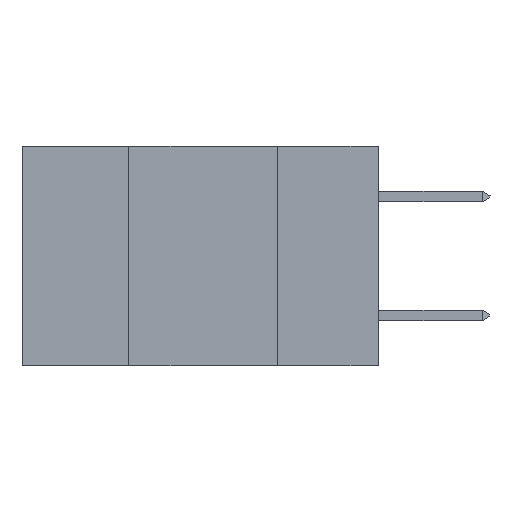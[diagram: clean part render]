
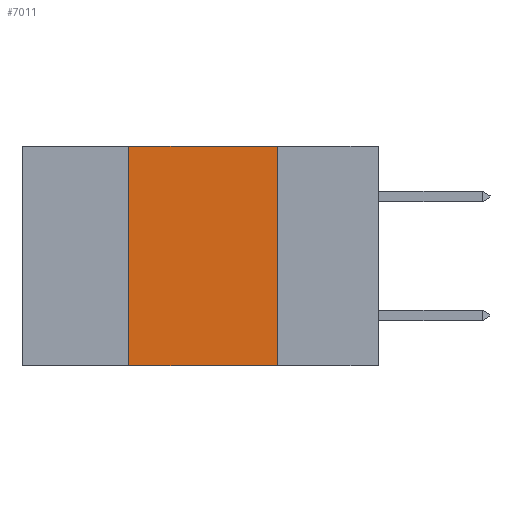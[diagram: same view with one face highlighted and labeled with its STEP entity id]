
A CAD part, left-side view. The second image highlights one B-rep face of the part: STEP entity #7011.
In plain terms, the highlighted planar face has unit normal (-1, 0, 0).
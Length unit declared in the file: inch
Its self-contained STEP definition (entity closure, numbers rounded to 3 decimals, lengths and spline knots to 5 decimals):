
#756 = CARTESIAN_POINT ( 'NONE',  ( 0., 0.17, 0. ) ) ;
#843 = AXIS2_PLACEMENT_3D ( 'NONE', #12461, #4452, #17508 ) ;
#1350 = LINE ( 'NONE', #20598, #4529 ) ;
#2626 = ORIENTED_EDGE ( 'NONE', *, *, #4256, .F. ) ;
#3302 = CARTESIAN_POINT ( 'NONE',  ( 0., 0.17, -0.37 ) ) ;
#3910 = VERTEX_POINT ( 'NONE', #6780 ) ;
#4190 = CARTESIAN_POINT ( 'NONE',  ( 0., 0.6, 0. ) ) ;
#4256 = EDGE_CURVE ( 'NONE', #8670, #11378, #6463, .T. ) ;
#4452 = DIRECTION ( 'NONE',  ( 1., 0., 0. ) ) ;
#4529 = VECTOR ( 'NONE', #16399, 39.37008 ) ;
#4582 = CARTESIAN_POINT ( 'NONE',  ( 0., 0.17, -0.37 ) ) ;
#5583 = DIRECTION ( 'NONE',  ( 0., -1., 0. ) ) ;
#6463 = LINE ( 'NONE', #3302, #13963 ) ;
#6780 = CARTESIAN_POINT ( 'NONE',  ( 0., 0.42, -0.37 ) ) ;
#7011 = ADVANCED_FACE ( 'NONE', ( #15941 ), #10862, .F. ) ;
#7565 = ORIENTED_EDGE ( 'NONE', *, *, #10920, .F. ) ;
#8507 = LINE ( 'NONE', #8926, #17499 ) ;
#8670 = VERTEX_POINT ( 'NONE', #756 ) ;
#8926 = CARTESIAN_POINT ( 'NONE',  ( 0., 0.6, -0.37 ) ) ;
#10862 = PLANE ( 'NONE',  #843 ) ;
#10920 = EDGE_CURVE ( 'NONE', #3910, #11398, #1350, .T. ) ;
#11055 = ORIENTED_EDGE ( 'NONE', *, *, #16998, .F. ) ;
#11378 = VERTEX_POINT ( 'NONE', #4582 ) ;
#11398 = VERTEX_POINT ( 'NONE', #17906 ) ;
#12461 = CARTESIAN_POINT ( 'NONE',  ( 0., 0.6, 0. ) ) ;
#13349 = DIRECTION ( 'NONE',  ( 0., -1., 0. ) ) ;
#13560 = LINE ( 'NONE', #4190, #18172 ) ;
#13963 = VECTOR ( 'NONE', #16246, 39.37008 ) ;
#15941 = FACE_OUTER_BOUND ( 'NONE', #16281, .T. ) ;
#16246 = DIRECTION ( 'NONE',  ( 0., 0., -1. ) ) ;
#16281 = EDGE_LOOP ( 'NONE', ( #2626, #11055, #7565, #16557 ) ) ;
#16399 = DIRECTION ( 'NONE',  ( 0., 0., 1. ) ) ;
#16557 = ORIENTED_EDGE ( 'NONE', *, *, #17033, .T. ) ;
#16998 = EDGE_CURVE ( 'NONE', #11398, #8670, #13560, .T. ) ;
#17033 = EDGE_CURVE ( 'NONE', #3910, #11378, #8507, .T. ) ;
#17499 = VECTOR ( 'NONE', #13349, 39.37008 ) ;
#17508 = DIRECTION ( 'NONE',  ( 0., 0., -1. ) ) ;
#17906 = CARTESIAN_POINT ( 'NONE',  ( 0., 0.42, 0. ) ) ;
#18172 = VECTOR ( 'NONE', #5583, 39.37008 ) ;
#20598 = CARTESIAN_POINT ( 'NONE',  ( 0., 0.42, -0.37 ) ) ;
